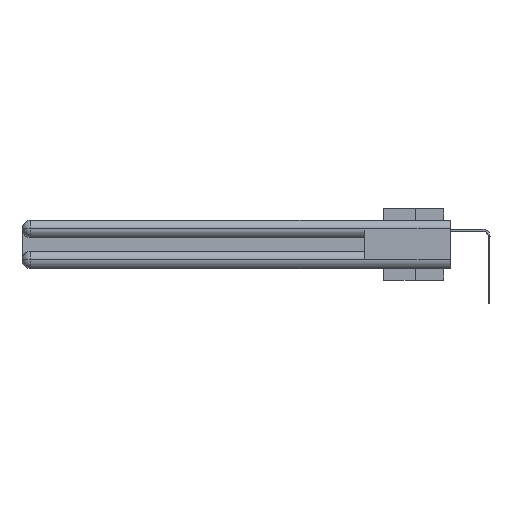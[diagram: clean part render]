
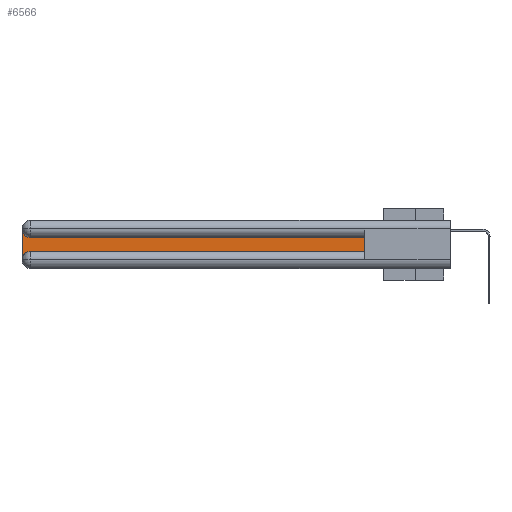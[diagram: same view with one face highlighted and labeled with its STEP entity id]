
A CAD part, left-side view. The second image highlights one B-rep face of the part: STEP entity #6566.
In plain terms, the highlighted planar face has unit normal (-1, 0, 0).
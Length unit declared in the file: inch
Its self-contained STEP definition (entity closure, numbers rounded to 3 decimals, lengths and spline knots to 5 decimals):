
#37 = DIRECTION ( 'NONE',  ( 1., 0., 0. ) ) ;
#195 = VECTOR ( 'NONE', #28663, 39.37008 ) ;
#453 = EDGE_CURVE ( 'NONE', #20983, #24550, #27079, .T. ) ;
#1124 = EDGE_CURVE ( 'NONE', #6427, #18334, #22585, .T. ) ;
#1909 = ORIENTED_EDGE ( 'NONE', *, *, #19646, .T. ) ;
#2391 = ORIENTED_EDGE ( 'NONE', *, *, #1124, .T. ) ;
#3082 = CARTESIAN_POINT ( 'NONE',  ( 0.075, 2.94, -0.0625 ) ) ;
#3365 = AXIS2_PLACEMENT_3D ( 'NONE', #28819, #17027, #7729 ) ;
#3409 = ORIENTED_EDGE ( 'NONE', *, *, #26968, .T. ) ;
#3551 = CIRCLE ( 'NONE', #23240, 0.06 ) ;
#4253 = LINE ( 'NONE', #21532, #195 ) ;
#4518 = CARTESIAN_POINT ( 'NONE',  ( 0.075, 0.6, -0.2175 ) ) ;
#4832 = VECTOR ( 'NONE', #16848, 39.37008 ) ;
#5021 = CARTESIAN_POINT ( 'NONE',  ( 0.075, 3., -0.1225 ) ) ;
#5717 = CIRCLE ( 'NONE', #3365, 0.06 ) ;
#6427 = VERTEX_POINT ( 'NONE', #23391 ) ;
#6566 = ADVANCED_FACE ( 'NONE', ( #7758 ), #7288, .F. ) ;
#6601 = CARTESIAN_POINT ( 'NONE',  ( 0.075, 0.6, -0.1225 ) ) ;
#7288 = PLANE ( 'NONE',  #27609 ) ;
#7439 = VERTEX_POINT ( 'NONE', #24887 ) ;
#7729 = DIRECTION ( 'NONE',  ( 0., 0., -1. ) ) ;
#7758 = FACE_OUTER_BOUND ( 'NONE', #12321, .T. ) ;
#7978 = DIRECTION ( 'NONE',  ( 1., 0., 0. ) ) ;
#9724 = CARTESIAN_POINT ( 'NONE',  ( 0.075, 3., -0.0625 ) ) ;
#10174 = ORIENTED_EDGE ( 'NONE', *, *, #453, .T. ) ;
#12321 = EDGE_LOOP ( 'NONE', ( #3409, #22197, #10174, #14604, #1909, #2391 ) ) ;
#13446 = CARTESIAN_POINT ( 'NONE',  ( 0.075, 3., -0.2175 ) ) ;
#13649 = DIRECTION ( 'NONE',  ( 0., 0., -1. ) ) ;
#13892 = LINE ( 'NONE', #4518, #19412 ) ;
#14582 = CARTESIAN_POINT ( 'NONE',  ( 0.075, 0.6, -0.2175 ) ) ;
#14604 = ORIENTED_EDGE ( 'NONE', *, *, #19770, .T. ) ;
#15980 = VECTOR ( 'NONE', #13649, 39.37008 ) ;
#16848 = DIRECTION ( 'NONE',  ( 0., 0., 1. ) ) ;
#17027 = DIRECTION ( 'NONE',  ( 1., 0., 0. ) ) ;
#18334 = VERTEX_POINT ( 'NONE', #6601 ) ;
#18983 = CARTESIAN_POINT ( 'NONE',  ( 0.075, 3., -0.2775 ) ) ;
#19412 = VECTOR ( 'NONE', #23427, 39.37008 ) ;
#19481 = VERTEX_POINT ( 'NONE', #25308 ) ;
#19561 = DIRECTION ( 'NONE',  ( 0., 0., -1. ) ) ;
#19646 = EDGE_CURVE ( 'NONE', #7439, #6427, #13892, .T. ) ;
#19770 = EDGE_CURVE ( 'NONE', #24550, #7439, #5717, .T. ) ;
#20983 = VERTEX_POINT ( 'NONE', #9724 ) ;
#21532 = CARTESIAN_POINT ( 'NONE',  ( 0.075, 0.6, -0.1225 ) ) ;
#22197 = ORIENTED_EDGE ( 'NONE', *, *, #25374, .T. ) ;
#22585 = LINE ( 'NONE', #14582, #4832 ) ;
#23240 = AXIS2_PLACEMENT_3D ( 'NONE', #3082, #7978, #19561 ) ;
#23391 = CARTESIAN_POINT ( 'NONE',  ( 0.075, 0.6, -0.2175 ) ) ;
#23427 = DIRECTION ( 'NONE',  ( 0., -1., 0. ) ) ;
#24550 = VERTEX_POINT ( 'NONE', #18983 ) ;
#24887 = CARTESIAN_POINT ( 'NONE',  ( 0.075, 2.94, -0.2175 ) ) ;
#25308 = CARTESIAN_POINT ( 'NONE',  ( 0.075, 2.94, -0.1225 ) ) ;
#25374 = EDGE_CURVE ( 'NONE', #19481, #20983, #3551, .T. ) ;
#26968 = EDGE_CURVE ( 'NONE', #18334, #19481, #4253, .T. ) ;
#27079 = LINE ( 'NONE', #13446, #15980 ) ;
#27609 = AXIS2_PLACEMENT_3D ( 'NONE', #5021, #37, #30673 ) ;
#28663 = DIRECTION ( 'NONE',  ( 0., 1., 0. ) ) ;
#28819 = CARTESIAN_POINT ( 'NONE',  ( 0.075, 2.94, -0.2775 ) ) ;
#30673 = DIRECTION ( 'NONE',  ( 0., 0., -1. ) ) ;
